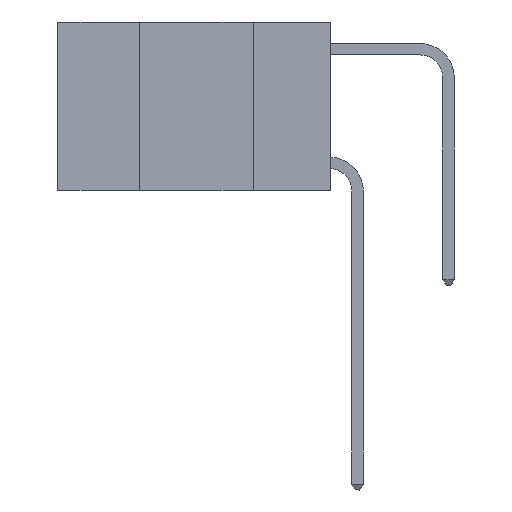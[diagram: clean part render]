
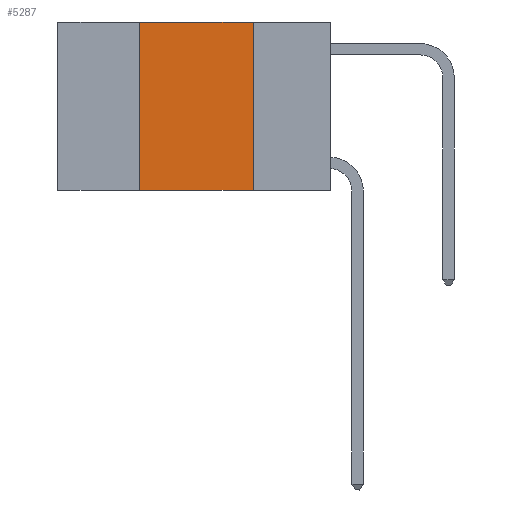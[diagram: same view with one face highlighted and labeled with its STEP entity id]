
A CAD part, left-side view. The second image highlights one B-rep face of the part: STEP entity #5287.
In plain terms, the highlighted planar face has unit normal (-1, 0, 0).
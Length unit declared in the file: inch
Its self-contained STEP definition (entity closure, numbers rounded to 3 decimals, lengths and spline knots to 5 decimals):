
#152 = CARTESIAN_POINT ( 'NONE',  ( 0., 0.6, 0. ) ) ;
#610 = LINE ( 'NONE', #11136, #7814 ) ;
#1715 = CARTESIAN_POINT ( 'NONE',  ( 0., 0.17, 0. ) ) ;
#1804 = CARTESIAN_POINT ( 'NONE',  ( 0., 0.6, 0. ) ) ;
#1970 = VECTOR ( 'NONE', #5952, 39.37008 ) ;
#2360 = ORIENTED_EDGE ( 'NONE', *, *, #3385, .F. ) ;
#2573 = ORIENTED_EDGE ( 'NONE', *, *, #2624, .F. ) ;
#2624 = EDGE_CURVE ( 'NONE', #12066, #4462, #13794, .T. ) ;
#2768 = CARTESIAN_POINT ( 'NONE',  ( 0., 0.42, 0. ) ) ;
#3385 = EDGE_CURVE ( 'NONE', #8223, #6045, #7433, .T. ) ;
#3716 = PLANE ( 'NONE',  #6205 ) ;
#4379 = CARTESIAN_POINT ( 'NONE',  ( 0., 0.42, 0. ) ) ;
#4462 = VERTEX_POINT ( 'NONE', #2768 ) ;
#4618 = EDGE_CURVE ( 'NONE', #4462, #8223, #10833, .T. ) ;
#5287 = ADVANCED_FACE ( 'NONE', ( #7802 ), #3716, .F. ) ;
#5387 = ORIENTED_EDGE ( 'NONE', *, *, #4618, .F. ) ;
#5396 = CARTESIAN_POINT ( 'NONE',  ( 0., 0.42, -0.37 ) ) ;
#5765 = EDGE_CURVE ( 'NONE', #12066, #6045, #610, .T. ) ;
#5952 = DIRECTION ( 'NONE',  ( 0., 0., 1. ) ) ;
#6045 = VERTEX_POINT ( 'NONE', #10921 ) ;
#6205 = AXIS2_PLACEMENT_3D ( 'NONE', #1804, #11422, #9294 ) ;
#6681 = EDGE_LOOP ( 'NONE', ( #2360, #5387, #2573, #12833 ) ) ;
#6785 = DIRECTION ( 'NONE',  ( 0., -1., 0. ) ) ;
#7433 = LINE ( 'NONE', #1715, #12854 ) ;
#7802 = FACE_OUTER_BOUND ( 'NONE', #6681, .T. ) ;
#7814 = VECTOR ( 'NONE', #6785, 39.37008 ) ;
#8223 = VERTEX_POINT ( 'NONE', #12150 ) ;
#8716 = DIRECTION ( 'NONE',  ( 0., -1., 0. ) ) ;
#9294 = DIRECTION ( 'NONE',  ( 0., 0., -1. ) ) ;
#10833 = LINE ( 'NONE', #152, #12743 ) ;
#10921 = CARTESIAN_POINT ( 'NONE',  ( 0., 0.17, -0.37 ) ) ;
#11136 = CARTESIAN_POINT ( 'NONE',  ( 0., 0.6, -0.37 ) ) ;
#11422 = DIRECTION ( 'NONE',  ( 1., 0., 0. ) ) ;
#12066 = VERTEX_POINT ( 'NONE', #5396 ) ;
#12150 = CARTESIAN_POINT ( 'NONE',  ( 0., 0.17, 0. ) ) ;
#12634 = DIRECTION ( 'NONE',  ( 0., 0., -1. ) ) ;
#12743 = VECTOR ( 'NONE', #8716, 39.37008 ) ;
#12833 = ORIENTED_EDGE ( 'NONE', *, *, #5765, .T. ) ;
#12854 = VECTOR ( 'NONE', #12634, 39.37008 ) ;
#13794 = LINE ( 'NONE', #4379, #1970 ) ;
